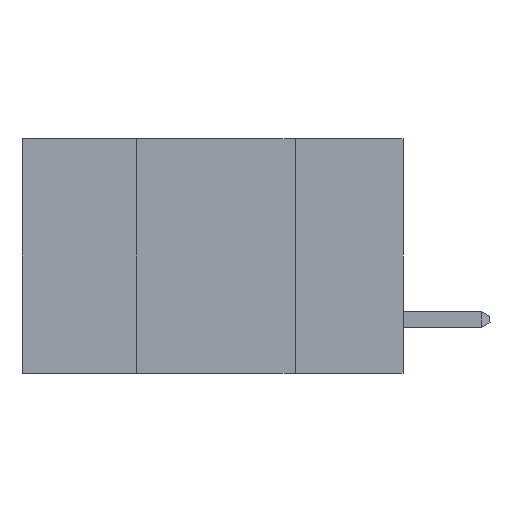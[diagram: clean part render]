
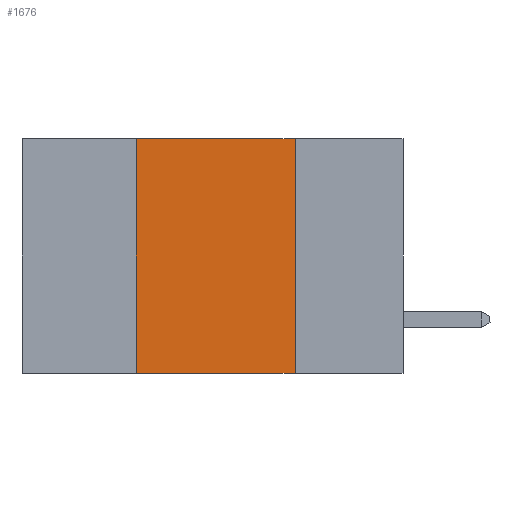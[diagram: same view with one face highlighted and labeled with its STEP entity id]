
A CAD part, left-side view. The second image highlights one B-rep face of the part: STEP entity #1676.
In plain terms, the highlighted planar face has unit normal (-1, 0, 0).
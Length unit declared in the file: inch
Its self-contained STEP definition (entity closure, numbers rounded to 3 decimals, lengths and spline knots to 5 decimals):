
#71 = DIRECTION ( 'NONE',  ( 0., 0., -1. ) ) ;
#235 = CARTESIAN_POINT ( 'NONE',  ( 0., 0.17, 0. ) ) ;
#277 = DIRECTION ( 'NONE',  ( 1., 0., 0. ) ) ;
#294 = DIRECTION ( 'NONE',  ( 0., 0., -1. ) ) ;
#739 = VERTEX_POINT ( 'NONE', #7185 ) ;
#942 = CARTESIAN_POINT ( 'NONE',  ( 0., 0.17, -0.37 ) ) ;
#1239 = VECTOR ( 'NONE', #71, 39.37008 ) ;
#1329 = VERTEX_POINT ( 'NONE', #942 ) ;
#1676 = ADVANCED_FACE ( 'NONE', ( #3535 ), #1956, .F. ) ;
#1893 = CARTESIAN_POINT ( 'NONE',  ( 0., 0.6, 0. ) ) ;
#1952 = AXIS2_PLACEMENT_3D ( 'NONE', #1893, #277, #294 ) ;
#1956 = PLANE ( 'NONE',  #1952 ) ;
#2061 = ORIENTED_EDGE ( 'NONE', *, *, #8092, .F. ) ;
#2106 = ORIENTED_EDGE ( 'NONE', *, *, #7792, .F. ) ;
#2145 = ORIENTED_EDGE ( 'NONE', *, *, #8346, .F. ) ;
#2195 = ORIENTED_EDGE ( 'NONE', *, *, #10107, .T. ) ;
#2644 = CARTESIAN_POINT ( 'NONE',  ( 0., 0.42, 0. ) ) ;
#2786 = VECTOR ( 'NONE', #10893, 39.37008 ) ;
#3472 = LINE ( 'NONE', #2644, #7805 ) ;
#3535 = FACE_OUTER_BOUND ( 'NONE', #8860, .T. ) ;
#3593 = VERTEX_POINT ( 'NONE', #235 ) ;
#3749 = DIRECTION ( 'NONE',  ( 0., -1., 0. ) ) ;
#3922 = LINE ( 'NONE', #5088, #1239 ) ;
#4552 = VERTEX_POINT ( 'NONE', #9990 ) ;
#5088 = CARTESIAN_POINT ( 'NONE',  ( 0., 0.17, 0. ) ) ;
#5499 = LINE ( 'NONE', #10354, #7699 ) ;
#7185 = CARTESIAN_POINT ( 'NONE',  ( 0., 0.42, -0.37 ) ) ;
#7699 = VECTOR ( 'NONE', #3749, 39.37008 ) ;
#7792 = EDGE_CURVE ( 'NONE', #4552, #3593, #5499, .T. ) ;
#7805 = VECTOR ( 'NONE', #7928, 39.37008 ) ;
#7928 = DIRECTION ( 'NONE',  ( 0., 0., 1. ) ) ;
#8092 = EDGE_CURVE ( 'NONE', #3593, #1329, #3922, .T. ) ;
#8346 = EDGE_CURVE ( 'NONE', #739, #4552, #3472, .T. ) ;
#8860 = EDGE_LOOP ( 'NONE', ( #2061, #2106, #2145, #2195 ) ) ;
#9599 = LINE ( 'NONE', #10088, #2786 ) ;
#9990 = CARTESIAN_POINT ( 'NONE',  ( 0., 0.42, 0. ) ) ;
#10088 = CARTESIAN_POINT ( 'NONE',  ( 0., 0.6, -0.37 ) ) ;
#10107 = EDGE_CURVE ( 'NONE', #739, #1329, #9599, .T. ) ;
#10354 = CARTESIAN_POINT ( 'NONE',  ( 0., 0.6, 0. ) ) ;
#10893 = DIRECTION ( 'NONE',  ( 0., -1., 0. ) ) ;
